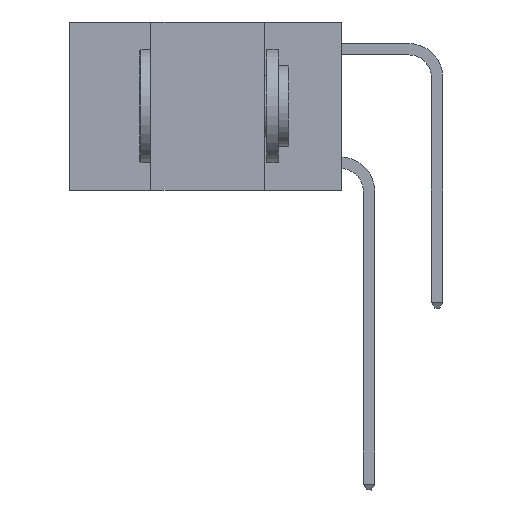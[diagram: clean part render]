
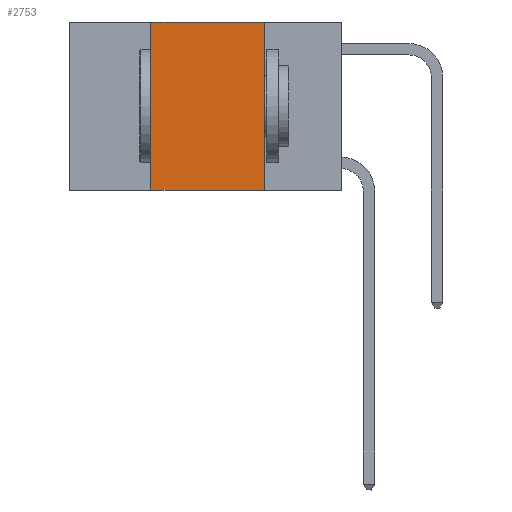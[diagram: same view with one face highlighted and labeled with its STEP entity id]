
A CAD part, left-side view. The second image highlights one B-rep face of the part: STEP entity #2753.
In plain terms, the highlighted planar face has unit normal (-1, 0, 0).
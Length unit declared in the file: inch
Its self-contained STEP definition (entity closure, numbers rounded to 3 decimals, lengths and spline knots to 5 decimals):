
#592 = CARTESIAN_POINT ( 'NONE',  ( 0., 0.17, -0.37 ) ) ;
#594 = CARTESIAN_POINT ( 'NONE',  ( 0., 0.6, -0.37 ) ) ;
#746 = PLANE ( 'NONE',  #8831 ) ;
#1269 = FACE_OUTER_BOUND ( 'NONE', #12783, .T. ) ;
#1560 = ORIENTED_EDGE ( 'NONE', *, *, #14693, .F. ) ;
#1819 = ORIENTED_EDGE ( 'NONE', *, *, #10120, .F. ) ;
#1855 = DIRECTION ( 'NONE',  ( 0., 0., 1. ) ) ;
#2072 = DIRECTION ( 'NONE',  ( 1., 0., 0. ) ) ;
#2406 = ORIENTED_EDGE ( 'NONE', *, *, #7396, .F. ) ;
#2707 = ORIENTED_EDGE ( 'NONE', *, *, #11261, .T. ) ;
#2720 = DIRECTION ( 'NONE',  ( 0., 0., -1. ) ) ;
#2733 = VERTEX_POINT ( 'NONE', #592 ) ;
#2753 = ADVANCED_FACE ( 'NONE', ( #1269 ), #746, .F. ) ;
#2943 = VECTOR ( 'NONE', #16467, 39.37008 ) ;
#4230 = LINE ( 'NONE', #8086, #10879 ) ;
#4519 = VECTOR ( 'NONE', #1855, 39.37008 ) ;
#4588 = CARTESIAN_POINT ( 'NONE',  ( 0., 0.42, 0. ) ) ;
#5389 = VERTEX_POINT ( 'NONE', #14871 ) ;
#5582 = CARTESIAN_POINT ( 'NONE',  ( 0., 0.17, 0. ) ) ;
#5832 = VECTOR ( 'NONE', #11262, 39.37008 ) ;
#7193 = VERTEX_POINT ( 'NONE', #5582 ) ;
#7396 = EDGE_CURVE ( 'NONE', #5389, #8176, #8460, .T. ) ;
#7412 = CARTESIAN_POINT ( 'NONE',  ( 0., 0.6, 0. ) ) ;
#8086 = CARTESIAN_POINT ( 'NONE',  ( 0., 0.17, 0. ) ) ;
#8176 = VERTEX_POINT ( 'NONE', #10116 ) ;
#8460 = LINE ( 'NONE', #4588, #4519 ) ;
#8831 = AXIS2_PLACEMENT_3D ( 'NONE', #13773, #2072, #2720 ) ;
#9333 = LINE ( 'NONE', #594, #5832 ) ;
#10116 = CARTESIAN_POINT ( 'NONE',  ( 0., 0.42, 0. ) ) ;
#10120 = EDGE_CURVE ( 'NONE', #8176, #7193, #15632, .T. ) ;
#10879 = VECTOR ( 'NONE', #15851, 39.37008 ) ;
#11261 = EDGE_CURVE ( 'NONE', #5389, #2733, #9333, .T. ) ;
#11262 = DIRECTION ( 'NONE',  ( 0., -1., 0. ) ) ;
#12783 = EDGE_LOOP ( 'NONE', ( #1560, #1819, #2406, #2707 ) ) ;
#13773 = CARTESIAN_POINT ( 'NONE',  ( 0., 0.6, 0. ) ) ;
#14693 = EDGE_CURVE ( 'NONE', #7193, #2733, #4230, .T. ) ;
#14871 = CARTESIAN_POINT ( 'NONE',  ( 0., 0.42, -0.37 ) ) ;
#15632 = LINE ( 'NONE', #7412, #2943 ) ;
#15851 = DIRECTION ( 'NONE',  ( 0., 0., -1. ) ) ;
#16467 = DIRECTION ( 'NONE',  ( 0., -1., 0. ) ) ;
